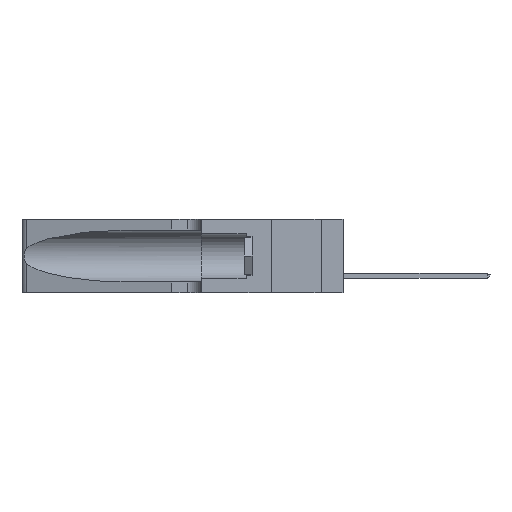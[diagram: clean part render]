
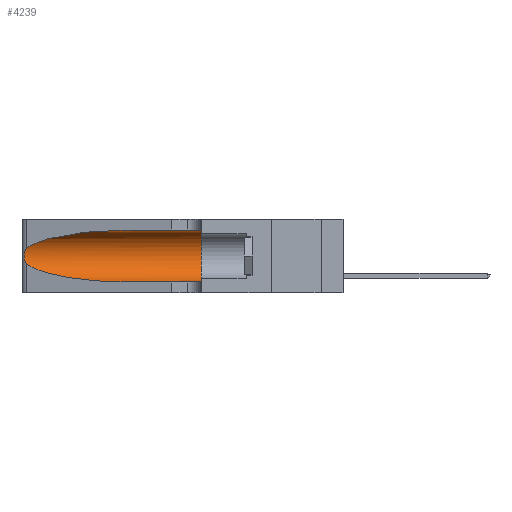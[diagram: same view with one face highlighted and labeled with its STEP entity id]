
A CAD part, left-side view. The second image highlights one B-rep face of the part: STEP entity #4239.
In plain terms, the highlighted cylindrical face has radius 3.308 mm (diameter 6.617 mm), a partial arc.
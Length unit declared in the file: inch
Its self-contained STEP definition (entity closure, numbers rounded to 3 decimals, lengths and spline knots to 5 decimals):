
#210 = VERTEX_POINT ( 'NONE', #7403 ) ;
#494 = CARTESIAN_POINT ( 'NONE',  ( 0.1305, 0.72297, 0.31525 ) ) ;
#647 = EDGE_CURVE ( 'NONE', #23923, #210, #11457, .T. ) ;
#984 = CARTESIAN_POINT ( 'NONE',  ( 0.26017, 1.23833, 0.17102 ) ) ;
#1059 = EDGE_LOOP ( 'NONE', ( #18339, #25821, #27640, #8262, #12373, #1725 ) ) ;
#1073 = DIRECTION ( 'NONE',  ( 0., 0., 1. ) ) ;
#1725 = ORIENTED_EDGE ( 'NONE', *, *, #22592, .F. ) ;
#2245 = EDGE_CURVE ( 'NONE', #13117, #23923, #2741, .T. ) ;
#2566 =( BOUNDED_CURVE ( )  B_SPLINE_CURVE ( 3, ( #18334, #14009, #13912, #24493 ),
 .UNSPECIFIED., .F., .F. ) 
 B_SPLINE_CURVE_WITH_KNOTS ( ( 4, 4 ),
 ( 3.44316, 4.71239 ),
 .UNSPECIFIED. ) 
 CURVE ( )  GEOMETRIC_REPRESENTATION_ITEM ( )  RATIONAL_B_SPLINE_CURVE ( ( 1., 0.87, 0.87, 1. ) ) 
 REPRESENTATION_ITEM ( '' )  );
#2741 =( BOUNDED_CURVE ( )  B_SPLINE_CURVE ( 3, ( #494, #15457, #7020, #26227 ),
 .UNSPECIFIED., .F., .T. ) 
 B_SPLINE_CURVE_WITH_KNOTS ( ( 4, 4 ),
 ( 1.5708, 2.84003 ),
 .UNSPECIFIED. ) 
 CURVE ( )  GEOMETRIC_REPRESENTATION_ITEM ( )  RATIONAL_B_SPLINE_CURVE ( ( 1., 0.87, 0.87, 1. ) ) 
 REPRESENTATION_ITEM ( '' )  );
#3157 = CARTESIAN_POINT ( 'NONE',  ( 0.25639, 1.23186, 0.15144 ) ) ;
#3629 = CARTESIAN_POINT ( 'NONE',  ( 0.1305, 0.72297, 0.31525 ) ) ;
#3772 = CARTESIAN_POINT ( 'NONE',  ( 0.1305, 1.61858, 0.31525 ) ) ;
#3916 = LINE ( 'NONE', #3772, #17308 ) ;
#4038 = DIRECTION ( 'NONE',  ( 0., -1., 0. ) ) ;
#4239 = ADVANCED_FACE ( 'NONE', ( #12659 ), #18389, .F. ) ;
#4914 = CARTESIAN_POINT ( 'NONE',  ( 0.25487, 1.22718, 0.22369 ) ) ;
#5287 = CARTESIAN_POINT ( 'NONE',  ( 0.25487, 1.22718, 0.14631 ) ) ;
#6628 = AXIS2_PLACEMENT_3D ( 'NONE', #17734, #9265, #8232 ) ;
#7018 = AXIS2_PLACEMENT_3D ( 'NONE', #9553, #22670, #1073 ) ;
#7020 = CARTESIAN_POINT ( 'NONE',  ( 0.2373, 1.15595, 0.28018 ) ) ;
#7195 = DIRECTION ( 'NONE',  ( 0., -1., 0. ) ) ;
#7217 = CARTESIAN_POINT ( 'NONE',  ( 0.25854, 1.2359, 0.20912 ) ) ;
#7403 = CARTESIAN_POINT ( 'NONE',  ( 0.25487, 1.22718, 0.14631 ) ) ;
#8232 = DIRECTION ( 'NONE',  ( 0., 0., -1. ) ) ;
#8262 = ORIENTED_EDGE ( 'NONE', *, *, #25088, .T. ) ;
#8307 = EDGE_CURVE ( 'NONE', #12871, #11930, #14949, .T. ) ;
#9144 = CARTESIAN_POINT ( 'NONE',  ( 0.1305, 1.61858, 0.05475 ) ) ;
#9169 = CARTESIAN_POINT ( 'NONE',  ( 0.25639, 1.23184, 0.21858 ) ) ;
#9265 = DIRECTION ( 'NONE',  ( 0., -1., 0. ) ) ;
#9553 = CARTESIAN_POINT ( 'NONE',  ( 0.1305, 0.35, 0.185 ) ) ;
#11457 = B_SPLINE_CURVE_WITH_KNOTS ( 'NONE', 3,
 ( #4914, #17838, #9169, #22035, #7217, #13507, #24453, #22129, #984, #15944, #22318, #3157, #18124, #5287 ),
 .UNSPECIFIED., .F., .F.,
 ( 4, 2, 2, 2, 2, 2, 4 ),
 ( 0., 0.00027, 0.00053, 0.00107, 0.0016, 0.00187, 0.00214 ),
 .UNSPECIFIED. ) ;
#11930 = VERTEX_POINT ( 'NONE', #21920 ) ;
#12373 = ORIENTED_EDGE ( 'NONE', *, *, #8307, .F. ) ;
#12491 = LINE ( 'NONE', #9144, #25254 ) ;
#12659 = FACE_OUTER_BOUND ( 'NONE', #1059, .T. ) ;
#12871 = VERTEX_POINT ( 'NONE', #17091 ) ;
#13117 = VERTEX_POINT ( 'NONE', #3629 ) ;
#13507 = CARTESIAN_POINT ( 'NONE',  ( 0.26018, 1.23835, 0.19895 ) ) ;
#13912 = CARTESIAN_POINT ( 'NONE',  ( 0.18966, 0.96281, 0.05475 ) ) ;
#14009 = CARTESIAN_POINT ( 'NONE',  ( 0.2373, 1.15595, 0.08982 ) ) ;
#14949 = CIRCLE ( 'NONE', #7018, 0.13025 ) ;
#15457 = CARTESIAN_POINT ( 'NONE',  ( 0.18966, 0.96281, 0.31525 ) ) ;
#15944 = CARTESIAN_POINT ( 'NONE',  ( 0.25856, 1.23593, 0.16098 ) ) ;
#16311 = VERTEX_POINT ( 'NONE', #27365 ) ;
#17091 = CARTESIAN_POINT ( 'NONE',  ( 0.1305, 0.35, 0.31525 ) ) ;
#17308 = VECTOR ( 'NONE', #4038, 39.37008 ) ;
#17448 = EDGE_CURVE ( 'NONE', #210, #16311, #2566, .T. ) ;
#17734 = CARTESIAN_POINT ( 'NONE',  ( 0.1305, 1.61858, 0.185 ) ) ;
#17838 = CARTESIAN_POINT ( 'NONE',  ( 0.25555, 1.22994, 0.2215 ) ) ;
#18124 = CARTESIAN_POINT ( 'NONE',  ( 0.25555, 1.22993, 0.14849 ) ) ;
#18334 = CARTESIAN_POINT ( 'NONE',  ( 0.25487, 1.22718, 0.14631 ) ) ;
#18339 = ORIENTED_EDGE ( 'NONE', *, *, #2245, .T. ) ;
#18389 = CYLINDRICAL_SURFACE ( 'NONE', #6628, 0.13025 ) ;
#21920 = CARTESIAN_POINT ( 'NONE',  ( 0.1305, 0.35, 0.05475 ) ) ;
#22035 = CARTESIAN_POINT ( 'NONE',  ( 0.25787, 1.23484, 0.2124 ) ) ;
#22129 = CARTESIAN_POINT ( 'NONE',  ( 0.26075, 1.23896, 0.178 ) ) ;
#22318 = CARTESIAN_POINT ( 'NONE',  ( 0.25789, 1.23486, 0.15765 ) ) ;
#22592 = EDGE_CURVE ( 'NONE', #13117, #12871, #3916, .T. ) ;
#22670 = DIRECTION ( 'NONE',  ( 0., 1., 0. ) ) ;
#23923 = VERTEX_POINT ( 'NONE', #25501 ) ;
#24453 = CARTESIAN_POINT ( 'NONE',  ( 0.26075, 1.23896, 0.19203 ) ) ;
#24493 = CARTESIAN_POINT ( 'NONE',  ( 0.1305, 0.72297, 0.05475 ) ) ;
#25088 = EDGE_CURVE ( 'NONE', #16311, #11930, #12491, .T. ) ;
#25254 = VECTOR ( 'NONE', #7195, 39.37008 ) ;
#25501 = CARTESIAN_POINT ( 'NONE',  ( 0.25487, 1.22718, 0.22369 ) ) ;
#25821 = ORIENTED_EDGE ( 'NONE', *, *, #647, .T. ) ;
#26227 = CARTESIAN_POINT ( 'NONE',  ( 0.25487, 1.22718, 0.22369 ) ) ;
#27365 = CARTESIAN_POINT ( 'NONE',  ( 0.1305, 0.72297, 0.05475 ) ) ;
#27640 = ORIENTED_EDGE ( 'NONE', *, *, #17448, .T. ) ;
